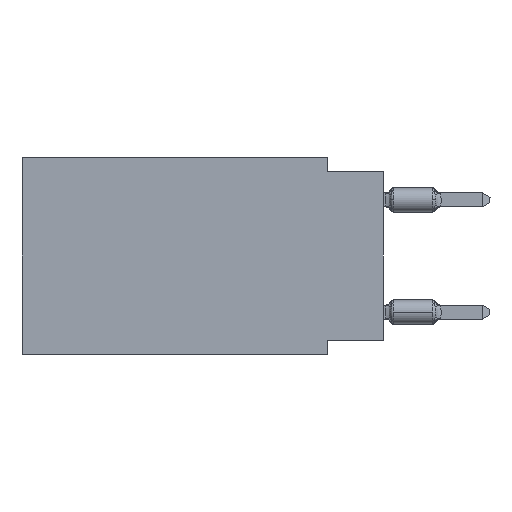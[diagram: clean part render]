
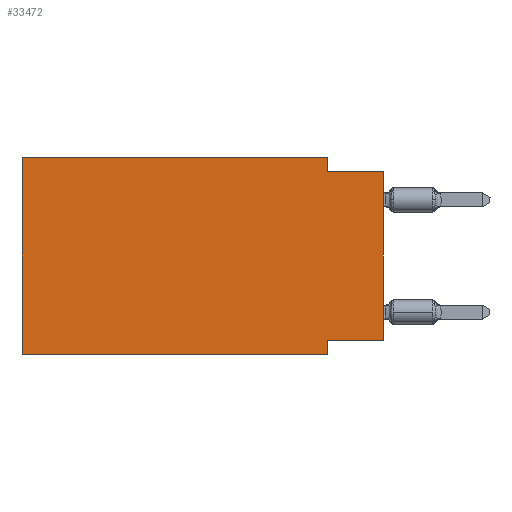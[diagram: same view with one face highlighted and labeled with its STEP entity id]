
A CAD part, left-side view. The second image highlights one B-rep face of the part: STEP entity #33472.
In plain terms, the highlighted planar face has unit normal (-1, 0, 0).
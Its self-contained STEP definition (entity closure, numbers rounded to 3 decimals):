
#369 = ORIENTED_EDGE ( 'NONE', *, *, #34889, .T. ) ;
#455 = ORIENTED_EDGE ( 'NONE', *, *, #8273, .F. ) ;
#1318 = ORIENTED_EDGE ( 'NONE', *, *, #16187, .F. ) ;
#1411 = ORIENTED_EDGE ( 'NONE', *, *, #36204, .F. ) ;
#3831 = ORIENTED_EDGE ( 'NONE', *, *, #21321, .F. ) ;
#4475 = VECTOR ( 'NONE', #4583, 1000. ) ;
#4583 = DIRECTION ( 'NONE',  ( 0., -1., 0. ) ) ;
#5742 = CARTESIAN_POINT ( 'NONE',  ( 0., 0., 0. ) ) ;
#6610 = VERTEX_POINT ( 'NONE', #33216 ) ;
#6901 = DIRECTION ( 'NONE',  ( 0., -1., 0. ) ) ;
#6983 = VECTOR ( 'NONE', #12688, 1000. ) ;
#7528 = VERTEX_POINT ( 'NONE', #25970 ) ;
#7554 = DIRECTION ( 'NONE',  ( 0., 1., 0. ) ) ;
#8019 = VERTEX_POINT ( 'NONE', #22602 ) ;
#8273 = EDGE_CURVE ( 'NONE', #26489, #9540, #11073, .T. ) ;
#8551 = PLANE ( 'NONE',  #35383 ) ;
#8705 = EDGE_LOOP ( 'NONE', ( #25538, #15135, #1411, #3831, #12253, #369, #1318, #455 ) ) ;
#9540 = VERTEX_POINT ( 'NONE', #22204 ) ;
#10741 = CARTESIAN_POINT ( 'NONE',  ( 0., 2.54, -0.635 ) ) ;
#10941 = DIRECTION ( 'NONE',  ( 0., 0., -1. ) ) ;
#11001 = CARTESIAN_POINT ( 'NONE',  ( 0., 16.383, 0. ) ) ;
#11073 = LINE ( 'NONE', #24605, #13662 ) ;
#11169 = CARTESIAN_POINT ( 'NONE',  ( 0., 16.383, 0. ) ) ;
#11682 = DIRECTION ( 'NONE',  ( 0., 0., 1. ) ) ;
#12247 = VECTOR ( 'NONE', #11682, 1000. ) ;
#12253 = ORIENTED_EDGE ( 'NONE', *, *, #24431, .F. ) ;
#12357 = VERTEX_POINT ( 'NONE', #36090 ) ;
#12688 = DIRECTION ( 'NONE',  ( 0., 0., 1. ) ) ;
#12760 = LINE ( 'NONE', #29974, #4475 ) ;
#13027 = CARTESIAN_POINT ( 'NONE',  ( 0., 16.383, -8.89 ) ) ;
#13662 = VECTOR ( 'NONE', #7554, 1000. ) ;
#14008 = VERTEX_POINT ( 'NONE', #11001 ) ;
#15135 = ORIENTED_EDGE ( 'NONE', *, *, #31351, .F. ) ;
#16023 = LINE ( 'NONE', #27314, #20073 ) ;
#16187 = EDGE_CURVE ( 'NONE', #9540, #12357, #30223, .T. ) ;
#16228 = EDGE_CURVE ( 'NONE', #26489, #6610, #22984, .T. ) ;
#16682 = CARTESIAN_POINT ( 'NONE',  ( 0., 2.54, -8.89 ) ) ;
#19489 = VERTEX_POINT ( 'NONE', #10741 ) ;
#19513 = DIRECTION ( 'NONE',  ( 1., 0., 0. ) ) ;
#20073 = VECTOR ( 'NONE', #29739, 1000. ) ;
#21321 = EDGE_CURVE ( 'NONE', #14008, #8019, #24200, .T. ) ;
#22204 = CARTESIAN_POINT ( 'NONE',  ( 0., 2.54, -8.255 ) ) ;
#22602 = CARTESIAN_POINT ( 'NONE',  ( 0., 2.54, 0. ) ) ;
#22919 = VECTOR ( 'NONE', #6901, 1000. ) ;
#22984 = LINE ( 'NONE', #5742, #12247 ) ;
#23620 = LINE ( 'NONE', #34952, #6983 ) ;
#24090 = CARTESIAN_POINT ( 'NONE',  ( 0., 0., -8.255 ) ) ;
#24200 = LINE ( 'NONE', #26420, #26026 ) ;
#24431 = EDGE_CURVE ( 'NONE', #7528, #14008, #23620, .T. ) ;
#24605 = CARTESIAN_POINT ( 'NONE',  ( 0., 0., -8.255 ) ) ;
#25048 = DIRECTION ( 'NONE',  ( 0., 0., -1. ) ) ;
#25538 = ORIENTED_EDGE ( 'NONE', *, *, #16228, .T. ) ;
#25970 = CARTESIAN_POINT ( 'NONE',  ( 0., 16.383, -8.89 ) ) ;
#26026 = VECTOR ( 'NONE', #29756, 1000. ) ;
#26420 = CARTESIAN_POINT ( 'NONE',  ( 0., 16.383, 0. ) ) ;
#26489 = VERTEX_POINT ( 'NONE', #24090 ) ;
#26916 = LINE ( 'NONE', #13027, #22919 ) ;
#27314 = CARTESIAN_POINT ( 'NONE',  ( 0., 2.54, 0. ) ) ;
#28203 = FACE_OUTER_BOUND ( 'NONE', #8705, .T. ) ;
#29739 = DIRECTION ( 'NONE',  ( 0., 0., -1. ) ) ;
#29756 = DIRECTION ( 'NONE',  ( 0., -1., 0. ) ) ;
#29974 = CARTESIAN_POINT ( 'NONE',  ( 0., 0., -0.635 ) ) ;
#30223 = LINE ( 'NONE', #16682, #35905 ) ;
#31351 = EDGE_CURVE ( 'NONE', #19489, #6610, #12760, .T. ) ;
#33216 = CARTESIAN_POINT ( 'NONE',  ( 0., 0., -0.635 ) ) ;
#33472 = ADVANCED_FACE ( 'NONE', ( #28203 ), #8551, .F. ) ;
#34889 = EDGE_CURVE ( 'NONE', #7528, #12357, #26916, .T. ) ;
#34952 = CARTESIAN_POINT ( 'NONE',  ( 0., 16.383, 0. ) ) ;
#35383 = AXIS2_PLACEMENT_3D ( 'NONE', #11169, #19513, #25048 ) ;
#35905 = VECTOR ( 'NONE', #10941, 1000. ) ;
#36090 = CARTESIAN_POINT ( 'NONE',  ( 0., 2.54, -8.89 ) ) ;
#36204 = EDGE_CURVE ( 'NONE', #8019, #19489, #16023, .T. ) ;
